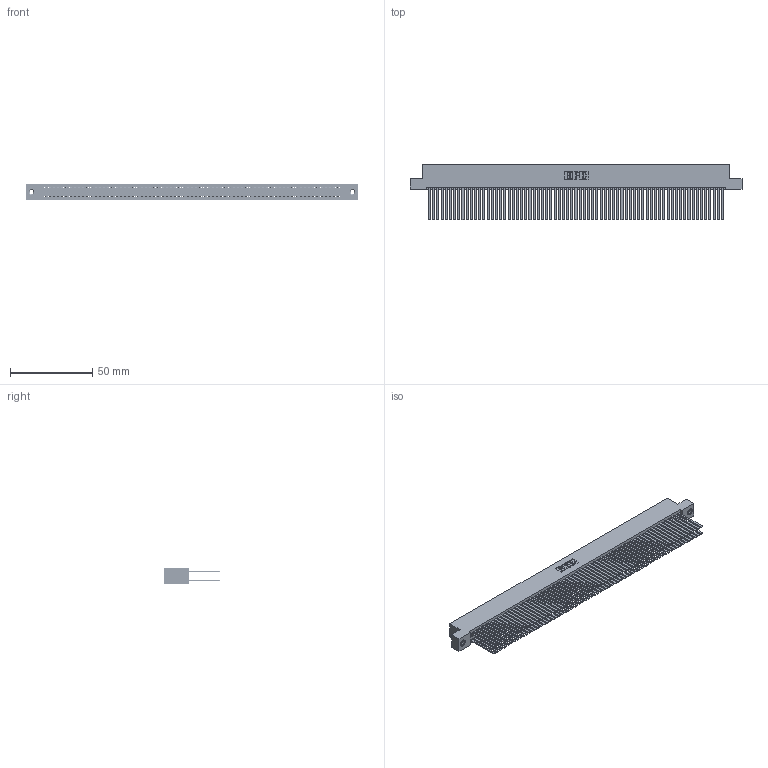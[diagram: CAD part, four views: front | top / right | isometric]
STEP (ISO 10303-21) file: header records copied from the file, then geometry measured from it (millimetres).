
FILE_DESCRIPTION (( 'STEP AP203' ), '1' );
FILE_NAME ('345-142-544-208.STEP', '2018-10-22T12:56:08', ( '' ), ( '' ), 'SwSTEP 2.0', 'SolidWorks 2016', '' );
FILE_SCHEMA (( 'CONFIG_CONTROL_DESIGN' ));
Length unit declared in the file: inch
Products named in the file (4): 345 Part_Flush Mounting Lugs - 0.156 Dia-TI; 345-292-001_345-293-144; 345-250-001_345-250-003-102; 345-142-544-208
Assembly tree (145 placements, depth 2):
  345-142-544-208
    345 Part_Flush Mounting Lugs - 0.156 Dia-TI
    345-292-001_345-293-144  x142
    345-250-001_345-250-003-102  x2
Bounding box: 201.55 x 33.96 x 9.4 mm (x, y, z)
Volume: 21831.9 mm3; surface area: 38680.6 mm2
Topology: 145 solids, 145 shells, 6434 faces, 19079 edges, 12522 vertices
Faces by surface type: plane 4230, cylinder 2188, cone 12, torus 4
Entity records: 52806 total; most frequent: CARTESIAN_POINT 8803, ORIENTED_EDGE 8730, DIRECTION 7751, EDGE_CURVE 4365, LINE 3933, VECTOR 3933, VERTEX_POINT 2904, AXIS2_PLACEMENT_3D 1909
